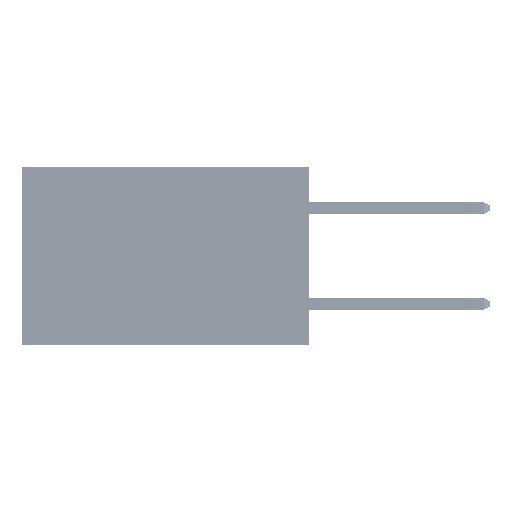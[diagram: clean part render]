
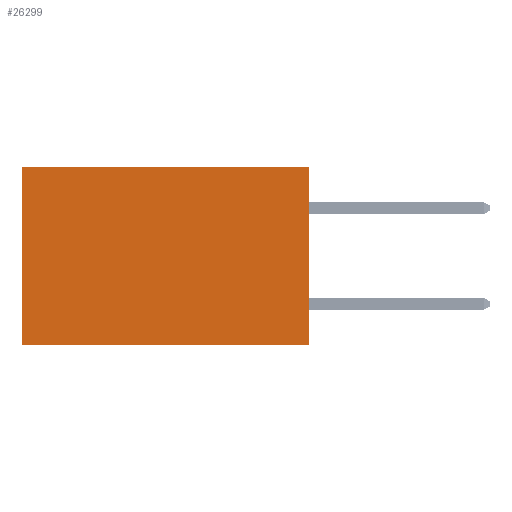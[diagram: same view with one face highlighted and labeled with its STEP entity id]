
A CAD part, left-side view. The second image highlights one B-rep face of the part: STEP entity #26299.
In plain terms, the highlighted planar face has unit normal (-1, 0, 0).
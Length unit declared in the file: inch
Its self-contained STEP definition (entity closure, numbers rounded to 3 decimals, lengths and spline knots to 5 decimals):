
#1442 = VERTEX_POINT ( 'NONE', #43287 ) ;
#3049 = CARTESIAN_POINT ( 'NONE',  ( 0.2875, 0., 0. ) ) ;
#3059 = ORIENTED_EDGE ( 'NONE', *, *, #14278, .T. ) ;
#4799 = VECTOR ( 'NONE', #27563, 39.37008 ) ;
#5180 = VERTEX_POINT ( 'NONE', #6507 ) ;
#6507 = CARTESIAN_POINT ( 'NONE',  ( 0.2875, 0.6, 0. ) ) ;
#7715 = CARTESIAN_POINT ( 'NONE',  ( 0.2875, 0., 0. ) ) ;
#8609 = CARTESIAN_POINT ( 'NONE',  ( 0.2875, 0.6, 0. ) ) ;
#9369 = ORIENTED_EDGE ( 'NONE', *, *, #47874, .F. ) ;
#10315 = VECTOR ( 'NONE', #36990, 39.37008 ) ;
#11169 = DIRECTION ( 'NONE',  ( 0., 0., -1. ) ) ;
#11572 = LINE ( 'NONE', #8609, #10315 ) ;
#13970 = ORIENTED_EDGE ( 'NONE', *, *, #42071, .F. ) ;
#14278 = EDGE_CURVE ( 'NONE', #41350, #5180, #30577, .T. ) ;
#18411 = CARTESIAN_POINT ( 'NONE',  ( 0.2875, 0., 0. ) ) ;
#18619 = CARTESIAN_POINT ( 'NONE',  ( 0.2875, 0., 0. ) ) ;
#19056 = EDGE_LOOP ( 'NONE', ( #22886, #9369, #13970, #3059 ) ) ;
#22149 = EDGE_CURVE ( 'NONE', #5180, #1442, #11572, .T. ) ;
#22291 = DIRECTION ( 'NONE',  ( 0., 1., 0. ) ) ;
#22641 = CARTESIAN_POINT ( 'NONE',  ( 0.2875, 0., -0.37 ) ) ;
#22886 = ORIENTED_EDGE ( 'NONE', *, *, #22149, .T. ) ;
#26299 = ADVANCED_FACE ( 'NONE', ( #36955 ), #31811, .F. ) ;
#27084 = CARTESIAN_POINT ( 'NONE',  ( 0.2875, 0., -0.37 ) ) ;
#27563 = DIRECTION ( 'NONE',  ( 0., 1., 0. ) ) ;
#30577 = LINE ( 'NONE', #18619, #4799 ) ;
#31811 = PLANE ( 'NONE',  #37699 ) ;
#32341 = LINE ( 'NONE', #22641, #39315 ) ;
#35907 = VERTEX_POINT ( 'NONE', #27084 ) ;
#36955 = FACE_OUTER_BOUND ( 'NONE', #19056, .T. ) ;
#36990 = DIRECTION ( 'NONE',  ( 0., 0., -1. ) ) ;
#37051 = LINE ( 'NONE', #3049, #37707 ) ;
#37699 = AXIS2_PLACEMENT_3D ( 'NONE', #7715, #44050, #48107 ) ;
#37707 = VECTOR ( 'NONE', #11169, 39.37008 ) ;
#39315 = VECTOR ( 'NONE', #22291, 39.37008 ) ;
#41350 = VERTEX_POINT ( 'NONE', #18411 ) ;
#42071 = EDGE_CURVE ( 'NONE', #41350, #35907, #37051, .T. ) ;
#43287 = CARTESIAN_POINT ( 'NONE',  ( 0.2875, 0.6, -0.37 ) ) ;
#44050 = DIRECTION ( 'NONE',  ( 1., 0., 0. ) ) ;
#47874 = EDGE_CURVE ( 'NONE', #35907, #1442, #32341, .T. ) ;
#48107 = DIRECTION ( 'NONE',  ( 0., 0., -1. ) ) ;
